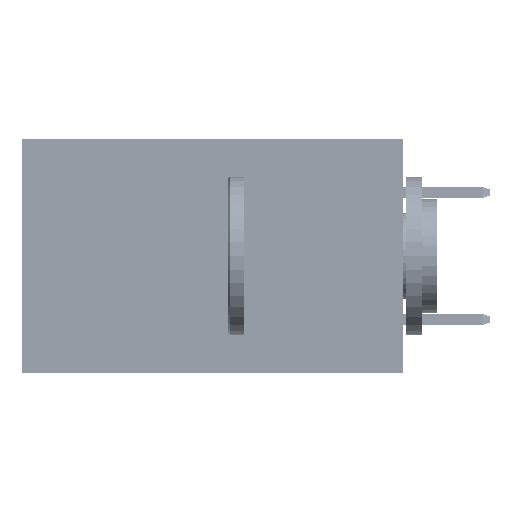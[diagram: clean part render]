
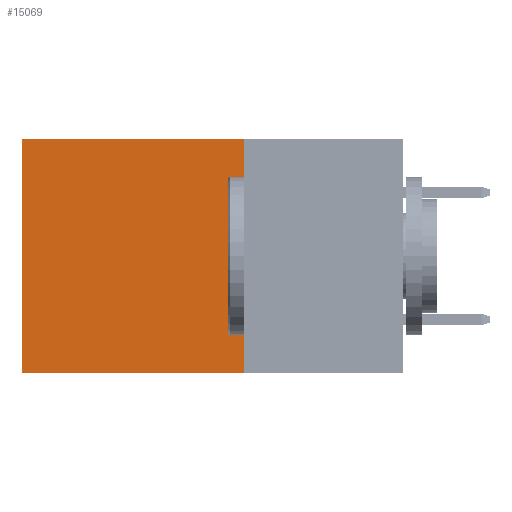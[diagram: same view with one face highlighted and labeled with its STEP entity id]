
A CAD part, left-side view. The second image highlights one B-rep face of the part: STEP entity #15069.
In plain terms, the highlighted planar face has unit normal (-1, 0, 0).
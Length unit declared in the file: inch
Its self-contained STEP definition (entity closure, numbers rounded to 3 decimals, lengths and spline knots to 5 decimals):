
#245 = CARTESIAN_POINT ( 'NONE',  ( 0.2875, 0.25, -0.37 ) ) ;
#1333 = VERTEX_POINT ( 'NONE', #9275 ) ;
#2223 = VERTEX_POINT ( 'NONE', #5433 ) ;
#3235 = EDGE_CURVE ( 'NONE', #2223, #46331, #11267, .T. ) ;
#3744 = DIRECTION ( 'NONE',  ( 0., 0., -1. ) ) ;
#4644 = ORIENTED_EDGE ( 'NONE', *, *, #11845, .F. ) ;
#5433 = CARTESIAN_POINT ( 'NONE',  ( 0.2875, 0.25, 0. ) ) ;
#6859 = CARTESIAN_POINT ( 'NONE',  ( 0.2875, 0.25, 0. ) ) ;
#6966 = LINE ( 'NONE', #13583, #31952 ) ;
#7635 = DIRECTION ( 'NONE',  ( 1., 0., 0. ) ) ;
#9275 = CARTESIAN_POINT ( 'NONE',  ( 0.2875, 0.6, -0.37 ) ) ;
#11118 = EDGE_CURVE ( 'NONE', #14185, #1333, #6966, .T. ) ;
#11267 = LINE ( 'NONE', #6859, #21504 ) ;
#11845 = EDGE_CURVE ( 'NONE', #46331, #1333, #27994, .T. ) ;
#12748 = AXIS2_PLACEMENT_3D ( 'NONE', #25941, #7635, #3744 ) ;
#13583 = CARTESIAN_POINT ( 'NONE',  ( 0.2875, 0.6, 0. ) ) ;
#14118 = VECTOR ( 'NONE', #34744, 39.37008 ) ;
#14185 = VERTEX_POINT ( 'NONE', #29589 ) ;
#15069 = ADVANCED_FACE ( 'NONE', ( #42699 ), #20633, .F. ) ;
#15579 = EDGE_CURVE ( 'NONE', #2223, #14185, #29460, .T. ) ;
#16055 = CARTESIAN_POINT ( 'NONE',  ( 0.2875, 0.25, -0.37 ) ) ;
#20131 = ORIENTED_EDGE ( 'NONE', *, *, #15579, .T. ) ;
#20633 = PLANE ( 'NONE',  #12748 ) ;
#21504 = VECTOR ( 'NONE', #32696, 39.37008 ) ;
#22060 = ORIENTED_EDGE ( 'NONE', *, *, #3235, .F. ) ;
#25941 = CARTESIAN_POINT ( 'NONE',  ( 0.2875, 0.25, 0. ) ) ;
#27994 = LINE ( 'NONE', #16055, #14118 ) ;
#29460 = LINE ( 'NONE', #44222, #34518 ) ;
#29589 = CARTESIAN_POINT ( 'NONE',  ( 0.2875, 0.6, 0. ) ) ;
#31952 = VECTOR ( 'NONE', #47602, 39.37008 ) ;
#32696 = DIRECTION ( 'NONE',  ( 0., 0., -1. ) ) ;
#33260 = ORIENTED_EDGE ( 'NONE', *, *, #11118, .T. ) ;
#34518 = VECTOR ( 'NONE', #36970, 39.37008 ) ;
#34744 = DIRECTION ( 'NONE',  ( 0., 1., 0. ) ) ;
#36970 = DIRECTION ( 'NONE',  ( 0., 1., 0. ) ) ;
#42539 = EDGE_LOOP ( 'NONE', ( #33260, #4644, #22060, #20131 ) ) ;
#42699 = FACE_OUTER_BOUND ( 'NONE', #42539, .T. ) ;
#44222 = CARTESIAN_POINT ( 'NONE',  ( 0.2875, 0.25, 0. ) ) ;
#46331 = VERTEX_POINT ( 'NONE', #245 ) ;
#47602 = DIRECTION ( 'NONE',  ( 0., 0., -1. ) ) ;
